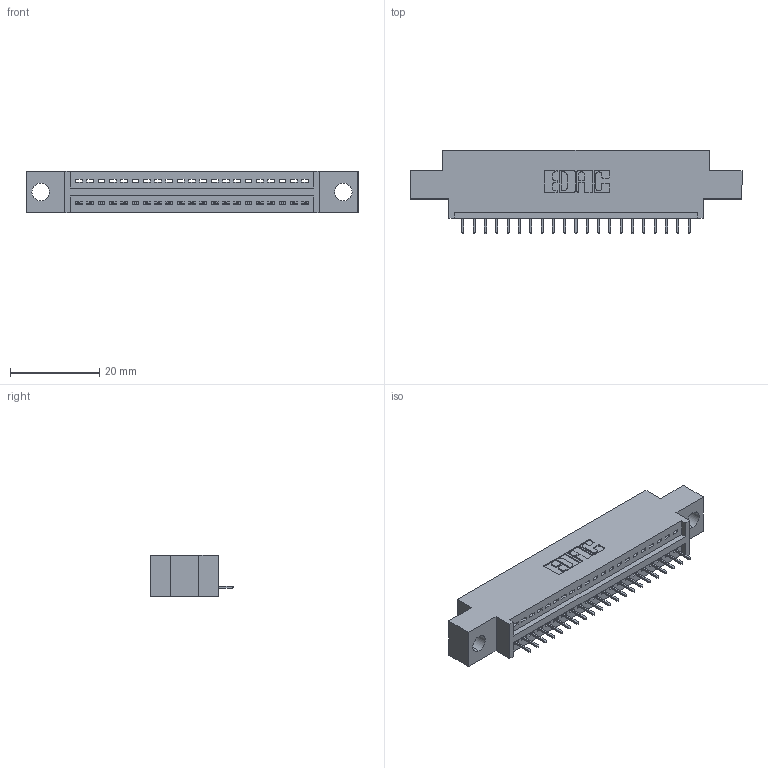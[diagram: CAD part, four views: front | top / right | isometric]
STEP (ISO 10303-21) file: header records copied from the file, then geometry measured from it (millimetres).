
FILE_DESCRIPTION (( 'STEP AP203' ), '1' );
FILE_NAME ('345-021-525-604.STEP', '2020-09-19T06:29:51', ( '' ), ( '' ), 'SwSTEP 2.0', 'SolidWorks 2020', '' );
FILE_SCHEMA (( 'CONFIG_CONTROL_DESIGN' ));
Length unit declared in the file: inch
Products named in the file (3): 345 Part_0.170 Offset - 0.156 Dia-TH; 345-021-525-604; 345-292-001_345-293-125
Assembly tree (22 placements, depth 2):
  345-021-525-604
    345 Part_0.170 Offset - 0.156 Dia-TH
    345-292-001_345-293-125  x21
Bounding box: 74.55 x 18.72 x 9.4 mm (x, y, z)
Volume: 6621.7 mm3; surface area: 8163.7 mm2
Topology: 22 solids, 22 shells, 1432 faces, 4133 edges, 2670 vertices
Faces by surface type: plane 1050, cylinder 382
Entity records: 18841 total; most frequent: CARTESIAN_POINT 3271, ORIENTED_EDGE 3226, DIRECTION 2887, EDGE_CURVE 1613, LINE 1401, VECTOR 1401, VERTEX_POINT 1070, AXIS2_PLACEMENT_3D 743
